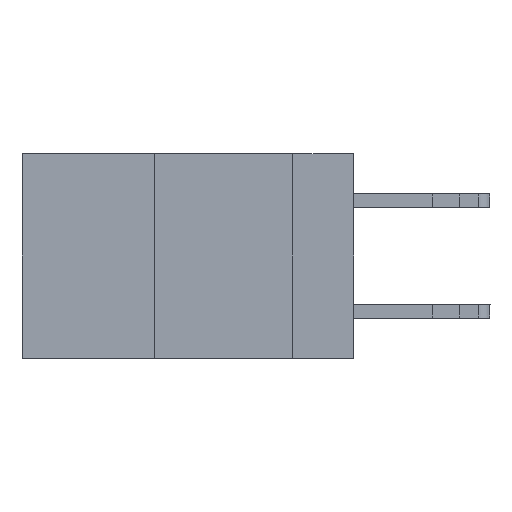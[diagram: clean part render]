
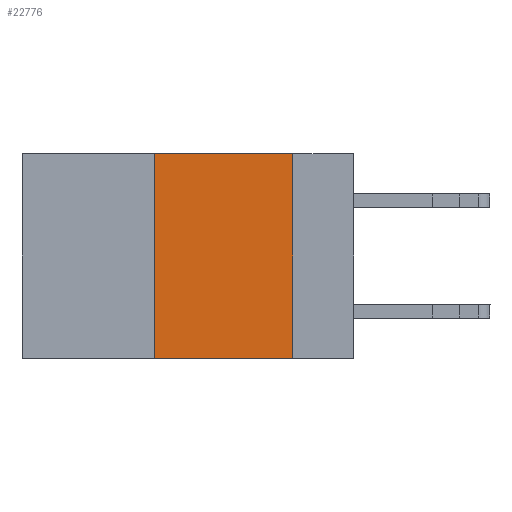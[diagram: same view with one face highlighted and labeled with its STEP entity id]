
A CAD part, left-side view. The second image highlights one B-rep face of the part: STEP entity #22776.
In plain terms, the highlighted planar face has unit normal (-1, 0, 0).
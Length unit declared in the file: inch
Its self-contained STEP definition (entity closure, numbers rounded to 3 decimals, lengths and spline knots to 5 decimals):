
#236 = DIRECTION ( 'NONE',  ( 0., 0., -1. ) ) ;
#800 = LINE ( 'NONE', #7852, #13462 ) ;
#2172 = VECTOR ( 'NONE', #10991, 39.37008 ) ;
#3644 = VECTOR ( 'NONE', #19563, 39.37008 ) ;
#4317 = ORIENTED_EDGE ( 'NONE', *, *, #18659, .T. ) ;
#5166 = EDGE_CURVE ( 'NONE', #23784, #10618, #5803, .T. ) ;
#5803 = LINE ( 'NONE', #8010, #27773 ) ;
#7852 = CARTESIAN_POINT ( 'NONE',  ( 0., 0.11, 0. ) ) ;
#8010 = CARTESIAN_POINT ( 'NONE',  ( 0., 0.36, 0. ) ) ;
#10091 = ORIENTED_EDGE ( 'NONE', *, *, #19761, .F. ) ;
#10618 = VERTEX_POINT ( 'NONE', #16945 ) ;
#10991 = DIRECTION ( 'NONE',  ( 0., -1., 0. ) ) ;
#11216 = CARTESIAN_POINT ( 'NONE',  ( 0., 0.36, -0.37 ) ) ;
#11629 = ORIENTED_EDGE ( 'NONE', *, *, #21722, .F. ) ;
#12161 = VERTEX_POINT ( 'NONE', #26623 ) ;
#13462 = VECTOR ( 'NONE', #23719, 39.37008 ) ;
#13593 = FACE_OUTER_BOUND ( 'NONE', #20322, .T. ) ;
#15279 = CARTESIAN_POINT ( 'NONE',  ( 0., 0.6, 0. ) ) ;
#15404 = LINE ( 'NONE', #22318, #2172 ) ;
#16945 = CARTESIAN_POINT ( 'NONE',  ( 0., 0.36, 0. ) ) ;
#17621 = LINE ( 'NONE', #15279, #3644 ) ;
#18165 = PLANE ( 'NONE',  #27589 ) ;
#18659 = EDGE_CURVE ( 'NONE', #23784, #12161, #15404, .T. ) ;
#19563 = DIRECTION ( 'NONE',  ( 0., -1., 0. ) ) ;
#19761 = EDGE_CURVE ( 'NONE', #28643, #12161, #800, .T. ) ;
#20322 = EDGE_LOOP ( 'NONE', ( #10091, #11629, #24579, #4317 ) ) ;
#20359 = DIRECTION ( 'NONE',  ( 1., 0., 0. ) ) ;
#21722 = EDGE_CURVE ( 'NONE', #10618, #28643, #17621, .T. ) ;
#22318 = CARTESIAN_POINT ( 'NONE',  ( 0., 0.6, -0.37 ) ) ;
#22776 = ADVANCED_FACE ( 'NONE', ( #13593 ), #18165, .F. ) ;
#23719 = DIRECTION ( 'NONE',  ( 0., 0., -1. ) ) ;
#23784 = VERTEX_POINT ( 'NONE', #11216 ) ;
#24579 = ORIENTED_EDGE ( 'NONE', *, *, #5166, .F. ) ;
#24937 = CARTESIAN_POINT ( 'NONE',  ( 0., 0.6, 0. ) ) ;
#25407 = CARTESIAN_POINT ( 'NONE',  ( 0., 0.11, 0. ) ) ;
#25798 = DIRECTION ( 'NONE',  ( 0., 0., 1. ) ) ;
#26623 = CARTESIAN_POINT ( 'NONE',  ( 0., 0.11, -0.37 ) ) ;
#27589 = AXIS2_PLACEMENT_3D ( 'NONE', #24937, #20359, #236 ) ;
#27773 = VECTOR ( 'NONE', #25798, 39.37008 ) ;
#28643 = VERTEX_POINT ( 'NONE', #25407 ) ;
